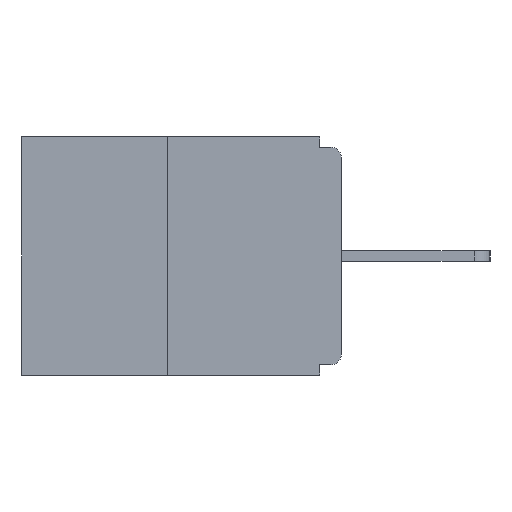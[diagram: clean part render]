
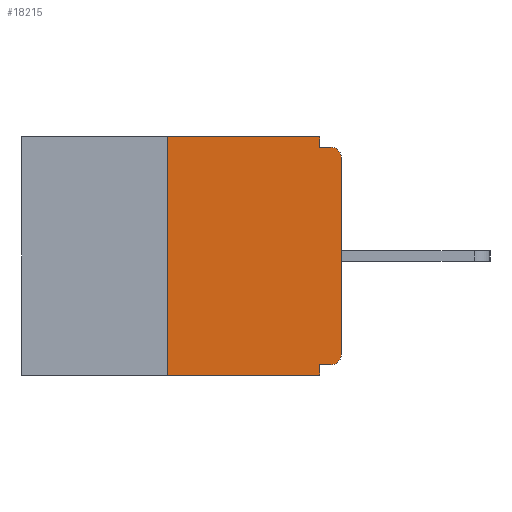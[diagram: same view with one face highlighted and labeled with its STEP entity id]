
A CAD part, left-side view. The second image highlights one B-rep face of the part: STEP entity #18215.
In plain terms, the highlighted planar face has unit normal (-1, 0, 0).
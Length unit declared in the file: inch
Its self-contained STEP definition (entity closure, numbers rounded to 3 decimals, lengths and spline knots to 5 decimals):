
#19 = VERTEX_POINT ( 'NONE', #9298 ) ;
#519 = AXIS2_PLACEMENT_3D ( 'NONE', #10748, #2002, #16038 ) ;
#542 = VERTEX_POINT ( 'NONE', #4655 ) ;
#555 = LINE ( 'NONE', #17905, #8275 ) ;
#688 = LINE ( 'NONE', #18149, #13084 ) ;
#807 = VECTOR ( 'NONE', #2979, 39.37008 ) ;
#979 = ORIENTED_EDGE ( 'NONE', *, *, #13529, .F. ) ;
#1254 = CIRCLE ( 'NONE', #519, 0.015 ) ;
#1457 = LINE ( 'NONE', #10330, #16893 ) ;
#1795 = VERTEX_POINT ( 'NONE', #22403 ) ;
#1977 = CARTESIAN_POINT ( 'NONE',  ( 0., 0., 0. ) ) ;
#2002 = DIRECTION ( 'NONE',  ( -1., 0., 0. ) ) ;
#2093 = LINE ( 'NONE', #1977, #19913 ) ;
#2290 = DIRECTION ( 'NONE',  ( -1., 0., 0. ) ) ;
#2788 = AXIS2_PLACEMENT_3D ( 'NONE', #16317, #2290, #17792 ) ;
#2979 = DIRECTION ( 'NONE',  ( 0., 1., 0. ) ) ;
#3047 = EDGE_CURVE ( 'NONE', #16489, #18002, #1457, .T. ) ;
#3119 = ORIENTED_EDGE ( 'NONE', *, *, #8872, .F. ) ;
#4474 = LINE ( 'NONE', #10093, #807 ) ;
#4655 = CARTESIAN_POINT ( 'NONE',  ( 0., 0., -0.313 ) ) ;
#4671 = VERTEX_POINT ( 'NONE', #20616 ) ;
#4831 = DIRECTION ( 'NONE',  ( 0., -1., 0. ) ) ;
#5058 = DIRECTION ( 'NONE',  ( 0., 0., -1. ) ) ;
#5303 = CARTESIAN_POINT ( 'NONE',  ( 0., 0.031, -0.015 ) ) ;
#6413 = FACE_OUTER_BOUND ( 'NONE', #21286, .T. ) ;
#7486 = CARTESIAN_POINT ( 'NONE',  ( 0., 0.25, 0. ) ) ;
#7553 = EDGE_CURVE ( 'NONE', #17840, #1795, #1254, .T. ) ;
#8272 = CARTESIAN_POINT ( 'NONE',  ( 0., 0.46, 0. ) ) ;
#8275 = VECTOR ( 'NONE', #12415, 39.37008 ) ;
#8390 = ORIENTED_EDGE ( 'NONE', *, *, #3047, .F. ) ;
#8872 = EDGE_CURVE ( 'NONE', #11769, #19, #9184, .T. ) ;
#9184 = LINE ( 'NONE', #19596, #22198 ) ;
#9298 = CARTESIAN_POINT ( 'NONE',  ( 0., 0.031, -0.343 ) ) ;
#9308 = EDGE_CURVE ( 'NONE', #10932, #16489, #688, .T. ) ;
#9360 = CARTESIAN_POINT ( 'NONE',  ( 0., 0.015, -0.328 ) ) ;
#9419 = CARTESIAN_POINT ( 'NONE',  ( 0., 0.25, 0. ) ) ;
#9466 = DIRECTION ( 'NONE',  ( 0., -1., 0. ) ) ;
#10093 = CARTESIAN_POINT ( 'NONE',  ( 0., 0., -0.328 ) ) ;
#10330 = CARTESIAN_POINT ( 'NONE',  ( 0., 0.031, 0. ) ) ;
#10349 = CARTESIAN_POINT ( 'NONE',  ( 0., 0.46, -0.343 ) ) ;
#10748 = CARTESIAN_POINT ( 'NONE',  ( 0., 0.015, -0.03 ) ) ;
#10838 = DIRECTION ( 'NONE',  ( 0., 0., 1. ) ) ;
#10932 = VERTEX_POINT ( 'NONE', #9419 ) ;
#11744 = LINE ( 'NONE', #10349, #11888 ) ;
#11769 = VERTEX_POINT ( 'NONE', #12674 ) ;
#11872 = VERTEX_POINT ( 'NONE', #9360 ) ;
#11888 = VECTOR ( 'NONE', #4831, 39.37008 ) ;
#12188 = ORIENTED_EDGE ( 'NONE', *, *, #16172, .T. ) ;
#12415 = DIRECTION ( 'NONE',  ( 0., -1., 0. ) ) ;
#12674 = CARTESIAN_POINT ( 'NONE',  ( 0., 0.031, -0.328 ) ) ;
#12704 = ORIENTED_EDGE ( 'NONE', *, *, #18004, .F. ) ;
#12945 = ORIENTED_EDGE ( 'NONE', *, *, #9308, .F. ) ;
#13084 = VECTOR ( 'NONE', #9466, 39.37008 ) ;
#13107 = LINE ( 'NONE', #7486, #15128 ) ;
#13420 = DIRECTION ( 'NONE',  ( 0., 0., -1. ) ) ;
#13529 = EDGE_CURVE ( 'NONE', #4671, #10932, #13107, .T. ) ;
#13772 = PLANE ( 'NONE',  #22180 ) ;
#14016 = EDGE_CURVE ( 'NONE', #11872, #11769, #4474, .T. ) ;
#14602 = DIRECTION ( 'NONE',  ( 0., 0., 1. ) ) ;
#15128 = VECTOR ( 'NONE', #14602, 39.37008 ) ;
#16038 = DIRECTION ( 'NONE',  ( 0., 0., -1. ) ) ;
#16172 = EDGE_CURVE ( 'NONE', #542, #17840, #2093, .T. ) ;
#16317 = CARTESIAN_POINT ( 'NONE',  ( 0., 0.015, -0.313 ) ) ;
#16460 = EDGE_CURVE ( 'NONE', #4671, #19, #11744, .T. ) ;
#16489 = VERTEX_POINT ( 'NONE', #19052 ) ;
#16893 = VECTOR ( 'NONE', #5058, 39.37008 ) ;
#17077 = ORIENTED_EDGE ( 'NONE', *, *, #17953, .T. ) ;
#17593 = ORIENTED_EDGE ( 'NONE', *, *, #7553, .T. ) ;
#17792 = DIRECTION ( 'NONE',  ( 0., 0., -1. ) ) ;
#17840 = VERTEX_POINT ( 'NONE', #19167 ) ;
#17905 = CARTESIAN_POINT ( 'NONE',  ( 0., 0., -0.015 ) ) ;
#17953 = EDGE_CURVE ( 'NONE', #11872, #542, #19623, .T. ) ;
#18002 = VERTEX_POINT ( 'NONE', #5303 ) ;
#18004 = EDGE_CURVE ( 'NONE', #18002, #1795, #555, .T. ) ;
#18149 = CARTESIAN_POINT ( 'NONE',  ( 0., 0.46, 0. ) ) ;
#18215 = ADVANCED_FACE ( 'NONE', ( #6413 ), #13772, .F. ) ;
#18289 = ORIENTED_EDGE ( 'NONE', *, *, #14016, .F. ) ;
#19052 = CARTESIAN_POINT ( 'NONE',  ( 0., 0.031, 0. ) ) ;
#19167 = CARTESIAN_POINT ( 'NONE',  ( 0., 0., -0.03 ) ) ;
#19596 = CARTESIAN_POINT ( 'NONE',  ( 0., 0.031, -0.343 ) ) ;
#19623 = CIRCLE ( 'NONE', #2788, 0.015 ) ;
#19819 = DIRECTION ( 'NONE',  ( 0., 0., -1. ) ) ;
#19913 = VECTOR ( 'NONE', #10838, 39.37008 ) ;
#20551 = ORIENTED_EDGE ( 'NONE', *, *, #16460, .T. ) ;
#20616 = CARTESIAN_POINT ( 'NONE',  ( 0., 0.25, -0.343 ) ) ;
#21286 = EDGE_LOOP ( 'NONE', ( #12945, #979, #20551, #3119, #18289, #17077, #12188, #17593, #12704, #8390 ) ) ;
#22121 = DIRECTION ( 'NONE',  ( 1., 0., 0. ) ) ;
#22180 = AXIS2_PLACEMENT_3D ( 'NONE', #8272, #22121, #13420 ) ;
#22198 = VECTOR ( 'NONE', #19819, 39.37008 ) ;
#22403 = CARTESIAN_POINT ( 'NONE',  ( 0., 0.015, -0.015 ) ) ;
